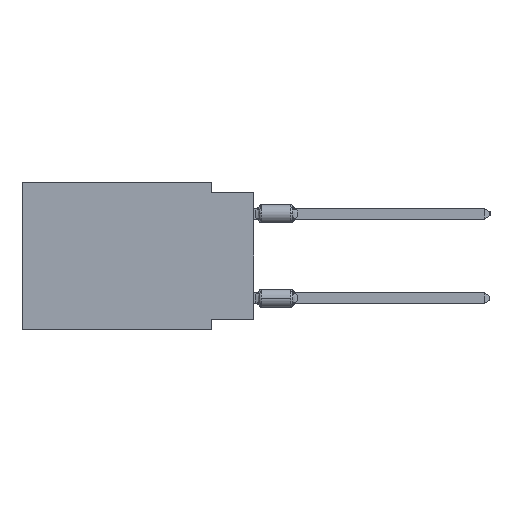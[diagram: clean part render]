
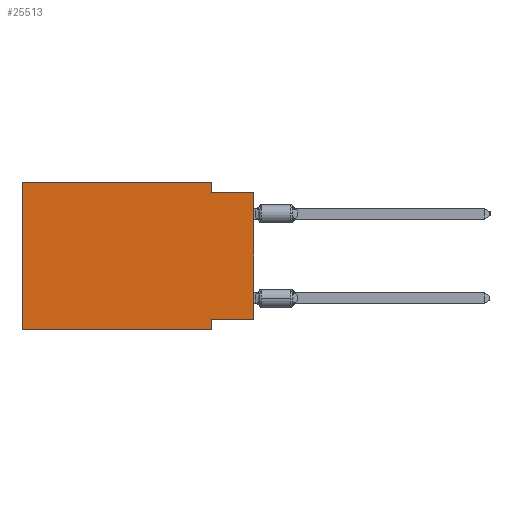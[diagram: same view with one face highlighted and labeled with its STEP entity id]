
A CAD part, left-side view. The second image highlights one B-rep face of the part: STEP entity #25513.
In plain terms, the highlighted planar face has unit normal (-1, 0, 0).
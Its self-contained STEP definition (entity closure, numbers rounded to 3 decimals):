
#286 = ORIENTED_EDGE ( 'NONE', *, *, #16802, .F. ) ;
#1169 = DIRECTION ( 'NONE',  ( 0., -1., 0. ) ) ;
#1240 = CARTESIAN_POINT ( 'NONE',  ( 0., 2.54, -0.635 ) ) ;
#1293 = EDGE_CURVE ( 'NONE', #26157, #7810, #15208, .T. ) ;
#1553 = CARTESIAN_POINT ( 'NONE',  ( 0., 2.54, -8.89 ) ) ;
#1837 = CARTESIAN_POINT ( 'NONE',  ( 0., 0., -8.255 ) ) ;
#2237 = DIRECTION ( 'NONE',  ( 0., 0., -1. ) ) ;
#3277 = VECTOR ( 'NONE', #14398, 1000. ) ;
#3883 = CARTESIAN_POINT ( 'NONE',  ( 0., 0., -0.635 ) ) ;
#5469 = DIRECTION ( 'NONE',  ( 0., 0., -1. ) ) ;
#6212 = DIRECTION ( 'NONE',  ( 0., -1., 0. ) ) ;
#7433 = VERTEX_POINT ( 'NONE', #34994 ) ;
#7810 = VERTEX_POINT ( 'NONE', #46965 ) ;
#8669 = EDGE_CURVE ( 'NONE', #46603, #26157, #15532, .T. ) ;
#9177 = LINE ( 'NONE', #3883, #38682 ) ;
#10381 = LINE ( 'NONE', #31062, #12936 ) ;
#10560 = DIRECTION ( 'NONE',  ( 0., 0., 1. ) ) ;
#11464 = DIRECTION ( 'NONE',  ( 1., 0., 0. ) ) ;
#11648 = EDGE_LOOP ( 'NONE', ( #35069, #286, #52916, #15252, #35712, #25865, #37457, #18542 ) ) ;
#12936 = VECTOR ( 'NONE', #1169, 1000. ) ;
#13119 = DIRECTION ( 'NONE',  ( 0., -1., 0. ) ) ;
#14398 = DIRECTION ( 'NONE',  ( 0., 0., -1. ) ) ;
#15120 = AXIS2_PLACEMENT_3D ( 'NONE', #23485, #11464, #2237 ) ;
#15208 = LINE ( 'NONE', #1553, #3277 ) ;
#15252 = ORIENTED_EDGE ( 'NONE', *, *, #19639, .F. ) ;
#15420 = LINE ( 'NONE', #24914, #15454 ) ;
#15454 = VECTOR ( 'NONE', #24076, 1000. ) ;
#15532 = LINE ( 'NONE', #1837, #29789 ) ;
#16802 = EDGE_CURVE ( 'NONE', #51815, #36886, #9177, .T. ) ;
#17896 = EDGE_CURVE ( 'NONE', #7433, #7810, #44475, .T. ) ;
#18542 = ORIENTED_EDGE ( 'NONE', *, *, #8669, .F. ) ;
#18681 = LINE ( 'NONE', #35690, #42712 ) ;
#19639 = EDGE_CURVE ( 'NONE', #27969, #35176, #10381, .T. ) ;
#19704 = DIRECTION ( 'NONE',  ( 0., 1., 0. ) ) ;
#23485 = CARTESIAN_POINT ( 'NONE',  ( 0., 13.97, 0. ) ) ;
#24076 = DIRECTION ( 'NONE',  ( 0., 0., 1. ) ) ;
#24914 = CARTESIAN_POINT ( 'NONE',  ( 0., 13.97, 0. ) ) ;
#25513 = ADVANCED_FACE ( 'NONE', ( #31583 ), #41041, .F. ) ;
#25865 = ORIENTED_EDGE ( 'NONE', *, *, #17896, .T. ) ;
#26157 = VERTEX_POINT ( 'NONE', #43276 ) ;
#27460 = CARTESIAN_POINT ( 'NONE',  ( 0., 13.97, -8.89 ) ) ;
#27969 = VERTEX_POINT ( 'NONE', #28956 ) ;
#28034 = VECTOR ( 'NONE', #6212, 1000. ) ;
#28763 = VECTOR ( 'NONE', #5469, 1000. ) ;
#28956 = CARTESIAN_POINT ( 'NONE',  ( 0., 13.97, 0. ) ) ;
#29789 = VECTOR ( 'NONE', #19704, 1000. ) ;
#31062 = CARTESIAN_POINT ( 'NONE',  ( 0., 13.97, 0. ) ) ;
#31583 = FACE_OUTER_BOUND ( 'NONE', #11648, .T. ) ;
#33142 = EDGE_CURVE ( 'NONE', #46603, #36886, #18681, .T. ) ;
#34802 = CARTESIAN_POINT ( 'NONE',  ( 0., 2.54, 0. ) ) ;
#34994 = CARTESIAN_POINT ( 'NONE',  ( 0., 13.97, -8.89 ) ) ;
#35069 = ORIENTED_EDGE ( 'NONE', *, *, #33142, .T. ) ;
#35176 = VERTEX_POINT ( 'NONE', #44309 ) ;
#35690 = CARTESIAN_POINT ( 'NONE',  ( 0., 0., 0. ) ) ;
#35712 = ORIENTED_EDGE ( 'NONE', *, *, #38221, .F. ) ;
#36886 = VERTEX_POINT ( 'NONE', #44774 ) ;
#37457 = ORIENTED_EDGE ( 'NONE', *, *, #1293, .F. ) ;
#38221 = EDGE_CURVE ( 'NONE', #7433, #27969, #15420, .T. ) ;
#38682 = VECTOR ( 'NONE', #13119, 1000. ) ;
#39419 = EDGE_CURVE ( 'NONE', #35176, #51815, #51838, .T. ) ;
#41041 = PLANE ( 'NONE',  #15120 ) ;
#42712 = VECTOR ( 'NONE', #10560, 1000. ) ;
#43276 = CARTESIAN_POINT ( 'NONE',  ( 0., 2.54, -8.255 ) ) ;
#44309 = CARTESIAN_POINT ( 'NONE',  ( 0., 2.54, 0. ) ) ;
#44475 = LINE ( 'NONE', #27460, #28034 ) ;
#44774 = CARTESIAN_POINT ( 'NONE',  ( 0., 0., -0.635 ) ) ;
#46603 = VERTEX_POINT ( 'NONE', #48816 ) ;
#46965 = CARTESIAN_POINT ( 'NONE',  ( 0., 2.54, -8.89 ) ) ;
#48816 = CARTESIAN_POINT ( 'NONE',  ( 0., 0., -8.255 ) ) ;
#51815 = VERTEX_POINT ( 'NONE', #1240 ) ;
#51838 = LINE ( 'NONE', #34802, #28763 ) ;
#52916 = ORIENTED_EDGE ( 'NONE', *, *, #39419, .F. ) ;
